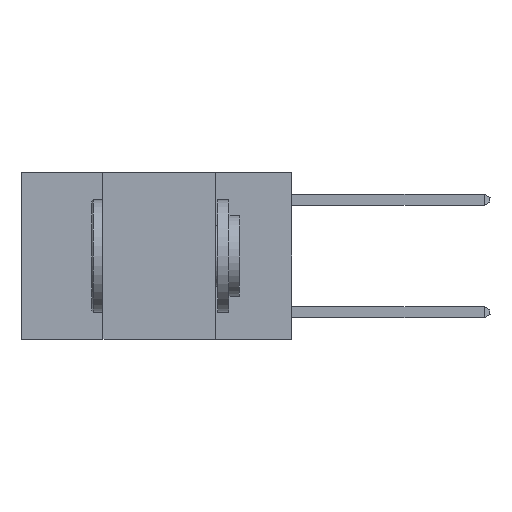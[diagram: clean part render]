
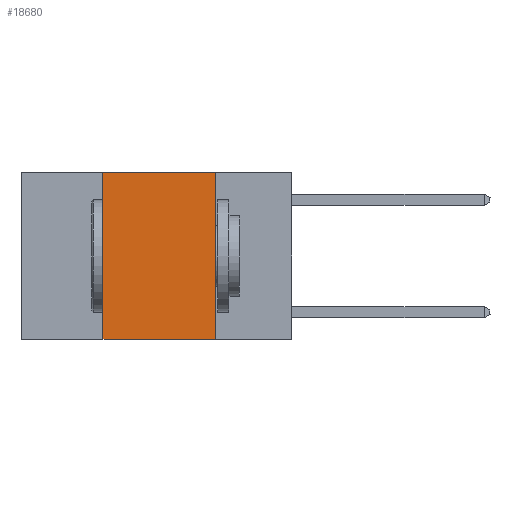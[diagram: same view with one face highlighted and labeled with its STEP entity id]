
A CAD part, left-side view. The second image highlights one B-rep face of the part: STEP entity #18680.
In plain terms, the highlighted planar face has unit normal (-1, 0, 0).
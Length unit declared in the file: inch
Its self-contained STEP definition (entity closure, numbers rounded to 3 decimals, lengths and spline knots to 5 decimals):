
#300 = LINE ( 'NONE', #7675, #12704 ) ;
#504 = LINE ( 'NONE', #9849, #8662 ) ;
#1226 = ORIENTED_EDGE ( 'NONE', *, *, #6910, .T. ) ;
#1564 = VECTOR ( 'NONE', #20776, 39.37008 ) ;
#1671 = PLANE ( 'NONE',  #8138 ) ;
#1904 = DIRECTION ( 'NONE',  ( 1., 0., 0. ) ) ;
#2439 = CARTESIAN_POINT ( 'NONE',  ( 0., 0.17, 0. ) ) ;
#3133 = EDGE_CURVE ( 'NONE', #14140, #9996, #300, .T. ) ;
#3487 = FACE_OUTER_BOUND ( 'NONE', #20688, .T. ) ;
#3883 = DIRECTION ( 'NONE',  ( 0., -1., 0. ) ) ;
#5826 = ORIENTED_EDGE ( 'NONE', *, *, #17939, .F. ) ;
#6397 = CARTESIAN_POINT ( 'NONE',  ( 0., 0.17, -0.37 ) ) ;
#6765 = CARTESIAN_POINT ( 'NONE',  ( 0., 0.42, 0. ) ) ;
#6910 = EDGE_CURVE ( 'NONE', #14140, #23031, #11173, .T. ) ;
#7675 = CARTESIAN_POINT ( 'NONE',  ( 0., 0.42, 0. ) ) ;
#8138 = AXIS2_PLACEMENT_3D ( 'NONE', #20122, #1904, #8828 ) ;
#8662 = VECTOR ( 'NONE', #22982, 39.37008 ) ;
#8828 = DIRECTION ( 'NONE',  ( 0., 0., -1. ) ) ;
#9543 = VECTOR ( 'NONE', #3883, 39.37008 ) ;
#9849 = CARTESIAN_POINT ( 'NONE',  ( 0., 0.6, 0. ) ) ;
#9996 = VERTEX_POINT ( 'NONE', #6765 ) ;
#11173 = LINE ( 'NONE', #16757, #9543 ) ;
#11617 = ORIENTED_EDGE ( 'NONE', *, *, #3133, .F. ) ;
#12369 = ORIENTED_EDGE ( 'NONE', *, *, #22338, .F. ) ;
#12704 = VECTOR ( 'NONE', #15082, 39.37008 ) ;
#14140 = VERTEX_POINT ( 'NONE', #15998 ) ;
#15082 = DIRECTION ( 'NONE',  ( 0., 0., 1. ) ) ;
#15998 = CARTESIAN_POINT ( 'NONE',  ( 0., 0.42, -0.37 ) ) ;
#16757 = CARTESIAN_POINT ( 'NONE',  ( 0., 0.6, -0.37 ) ) ;
#17067 = CARTESIAN_POINT ( 'NONE',  ( 0., 0.17, 0. ) ) ;
#17124 = LINE ( 'NONE', #2439, #1564 ) ;
#17939 = EDGE_CURVE ( 'NONE', #21284, #23031, #17124, .T. ) ;
#18680 = ADVANCED_FACE ( 'NONE', ( #3487 ), #1671, .F. ) ;
#20122 = CARTESIAN_POINT ( 'NONE',  ( 0., 0.6, 0. ) ) ;
#20688 = EDGE_LOOP ( 'NONE', ( #5826, #12369, #11617, #1226 ) ) ;
#20776 = DIRECTION ( 'NONE',  ( 0., 0., -1. ) ) ;
#21284 = VERTEX_POINT ( 'NONE', #17067 ) ;
#22338 = EDGE_CURVE ( 'NONE', #9996, #21284, #504, .T. ) ;
#22982 = DIRECTION ( 'NONE',  ( 0., -1., 0. ) ) ;
#23031 = VERTEX_POINT ( 'NONE', #6397 ) ;
